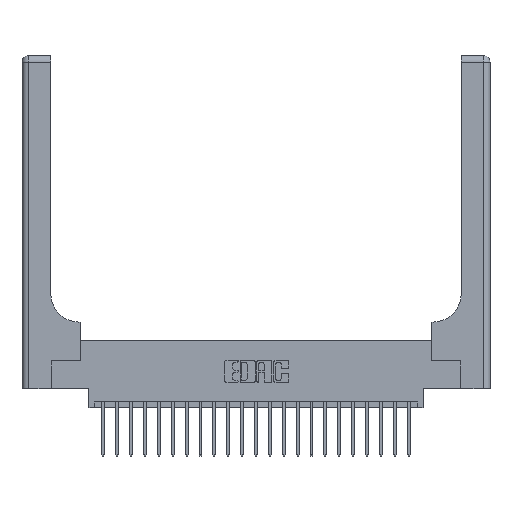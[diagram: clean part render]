
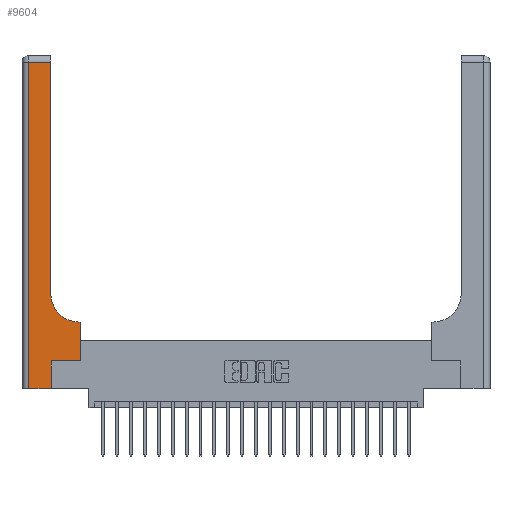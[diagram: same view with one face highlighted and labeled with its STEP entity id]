
A CAD part, top view. The second image highlights one B-rep face of the part: STEP entity #9604.
In plain terms, the highlighted planar face has unit normal (0, 0, 1).
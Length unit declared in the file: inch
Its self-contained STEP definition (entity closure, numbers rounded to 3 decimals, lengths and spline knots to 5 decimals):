
#128 = VECTOR ( 'NONE', #7702, 39.37008 ) ;
#165 = ORIENTED_EDGE ( 'NONE', *, *, #11328, .T. ) ;
#979 = DIRECTION ( 'NONE',  ( 1., 0., 0. ) ) ;
#1088 = CARTESIAN_POINT ( 'NONE',  ( 0., 3., 0.37 ) ) ;
#1092 = DIRECTION ( 'NONE',  ( 0., 1., 0. ) ) ;
#1442 = CARTESIAN_POINT ( 'NONE',  ( 0., 2.94, 0.37 ) ) ;
#2059 = LINE ( 'NONE', #20831, #10617 ) ;
#2603 = LINE ( 'NONE', #9479, #128 ) ;
#3837 = ORIENTED_EDGE ( 'NONE', *, *, #5797, .T. ) ;
#4166 = EDGE_CURVE ( 'NONE', #6861, #17297, #18102, .T. ) ;
#4289 = CARTESIAN_POINT ( 'NONE',  ( 0.528, 0.25, 0.37 ) ) ;
#4620 = CARTESIAN_POINT ( 'NONE',  ( 0.265, 0.25, 0.37 ) ) ;
#4798 = ORIENTED_EDGE ( 'NONE', *, *, #9004, .T. ) ;
#4877 = VERTEX_POINT ( 'NONE', #10627 ) ;
#5347 = DIRECTION ( 'NONE',  ( 0., 1., 0. ) ) ;
#5534 = VERTEX_POINT ( 'NONE', #15060 ) ;
#5663 = EDGE_CURVE ( 'NONE', #5534, #18133, #7826, .T. ) ;
#5797 = EDGE_CURVE ( 'NONE', #4877, #20735, #18340, .T. ) ;
#6649 = DIRECTION ( 'NONE',  ( 0., 0., -1. ) ) ;
#6774 = EDGE_CURVE ( 'NONE', #20735, #6861, #22488, .T. ) ;
#6861 = VERTEX_POINT ( 'NONE', #4289 ) ;
#7002 = CARTESIAN_POINT ( 'NONE',  ( 0.51, 0.85, 0.37 ) ) ;
#7620 = ORIENTED_EDGE ( 'NONE', *, *, #9805, .T. ) ;
#7702 = DIRECTION ( 'NONE',  ( -1., 0., 0. ) ) ;
#7826 = CIRCLE ( 'NONE', #13471, 0.25 ) ;
#8148 = CARTESIAN_POINT ( 'NONE',  ( 0.06, 2.94, 0.37 ) ) ;
#8438 = VERTEX_POINT ( 'NONE', #15172 ) ;
#8642 = LINE ( 'NONE', #14087, #19245 ) ;
#8777 = DIRECTION ( 'NONE',  ( -1., 0., 0. ) ) ;
#9004 = EDGE_CURVE ( 'NONE', #17297, #5534, #2603, .T. ) ;
#9479 = CARTESIAN_POINT ( 'NONE',  ( 0.26, 0.6, 0.37 ) ) ;
#9604 = ADVANCED_FACE ( 'NONE', ( #20705 ), #21933, .F. ) ;
#9805 = EDGE_CURVE ( 'NONE', #13307, #19920, #19641, .T. ) ;
#10019 = DIRECTION ( 'NONE',  ( 1., 0., 0. ) ) ;
#10480 = AXIS2_PLACEMENT_3D ( 'NONE', #1088, #15282, #21822 ) ;
#10617 = VECTOR ( 'NONE', #1092, 39.37008 ) ;
#10627 = CARTESIAN_POINT ( 'NONE',  ( 0.265, 0., 0.37 ) ) ;
#11328 = EDGE_CURVE ( 'NONE', #18133, #13307, #2059, .T. ) ;
#11393 = VECTOR ( 'NONE', #10019, 39.37008 ) ;
#11672 = ORIENTED_EDGE ( 'NONE', *, *, #20907, .T. ) ;
#12982 = ORIENTED_EDGE ( 'NONE', *, *, #6774, .T. ) ;
#13307 = VERTEX_POINT ( 'NONE', #20787 ) ;
#13471 = AXIS2_PLACEMENT_3D ( 'NONE', #7002, #6649, #22830 ) ;
#13913 = CARTESIAN_POINT ( 'NONE',  ( 0., 0., 0.37 ) ) ;
#14087 = CARTESIAN_POINT ( 'NONE',  ( 0.06, 3., 0.37 ) ) ;
#14181 = EDGE_LOOP ( 'NONE', ( #165, #7620, #11672, #20715, #3837, #12982, #14942, #4798, #19629 ) ) ;
#14451 = CARTESIAN_POINT ( 'NONE',  ( 0.528, 0.25, 0.37 ) ) ;
#14942 = ORIENTED_EDGE ( 'NONE', *, *, #4166, .T. ) ;
#15060 = CARTESIAN_POINT ( 'NONE',  ( 0.51, 0.6, 0.37 ) ) ;
#15172 = CARTESIAN_POINT ( 'NONE',  ( 0.06, 0., 0.37 ) ) ;
#15282 = DIRECTION ( 'NONE',  ( 0., 0., -1. ) ) ;
#15795 = LINE ( 'NONE', #13913, #11393 ) ;
#16101 = CARTESIAN_POINT ( 'NONE',  ( 0.265, 0., 0.37 ) ) ;
#16177 = EDGE_CURVE ( 'NONE', #8438, #4877, #15795, .T. ) ;
#17297 = VERTEX_POINT ( 'NONE', #22764 ) ;
#18089 = DIRECTION ( 'NONE',  ( 0., -1., 0. ) ) ;
#18102 = LINE ( 'NONE', #14451, #18313 ) ;
#18133 = VERTEX_POINT ( 'NONE', #18820 ) ;
#18313 = VECTOR ( 'NONE', #21645, 39.37008 ) ;
#18340 = LINE ( 'NONE', #16101, #22461 ) ;
#18820 = CARTESIAN_POINT ( 'NONE',  ( 0.26, 0.85, 0.37 ) ) ;
#19096 = VECTOR ( 'NONE', #8777, 39.37008 ) ;
#19245 = VECTOR ( 'NONE', #18089, 39.37008 ) ;
#19629 = ORIENTED_EDGE ( 'NONE', *, *, #5663, .T. ) ;
#19641 = LINE ( 'NONE', #1442, #19096 ) ;
#19920 = VERTEX_POINT ( 'NONE', #8148 ) ;
#20590 = CARTESIAN_POINT ( 'NONE',  ( 0.265, 0.25, 0.37 ) ) ;
#20705 = FACE_OUTER_BOUND ( 'NONE', #14181, .T. ) ;
#20715 = ORIENTED_EDGE ( 'NONE', *, *, #16177, .T. ) ;
#20735 = VERTEX_POINT ( 'NONE', #4620 ) ;
#20787 = CARTESIAN_POINT ( 'NONE',  ( 0.26, 2.94, 0.37 ) ) ;
#20831 = CARTESIAN_POINT ( 'NONE',  ( 0.26, 3., 0.37 ) ) ;
#20907 = EDGE_CURVE ( 'NONE', #19920, #8438, #8642, .T. ) ;
#21645 = DIRECTION ( 'NONE',  ( 0., 1., 0. ) ) ;
#21822 = DIRECTION ( 'NONE',  ( -1., 0., 0. ) ) ;
#21933 = PLANE ( 'NONE',  #10480 ) ;
#22461 = VECTOR ( 'NONE', #5347, 39.37008 ) ;
#22488 = LINE ( 'NONE', #20590, #22870 ) ;
#22764 = CARTESIAN_POINT ( 'NONE',  ( 0.528, 0.6, 0.37 ) ) ;
#22830 = DIRECTION ( 'NONE',  ( 1., 0., 0. ) ) ;
#22870 = VECTOR ( 'NONE', #979, 39.37008 ) ;
